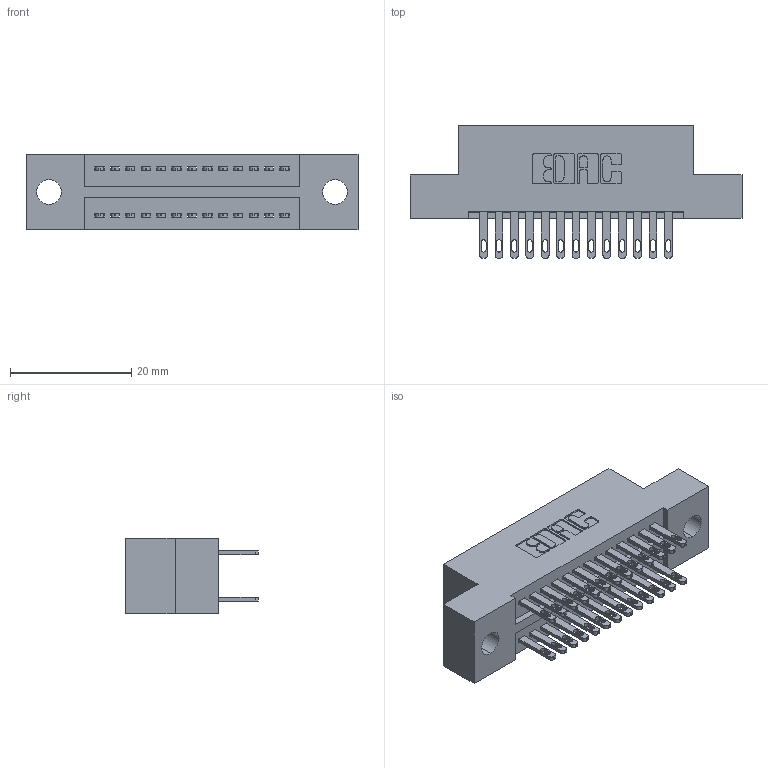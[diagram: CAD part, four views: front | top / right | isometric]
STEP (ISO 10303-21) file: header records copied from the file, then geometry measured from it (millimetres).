
FILE_DESCRIPTION (( 'STEP AP203' ), '1' );
FILE_NAME ('325-026-500-209.STEP', '2020-02-24T18:13:38', ( '' ), ( '' ), 'SwSTEP 2.0', 'SolidWorks 2016', '' );
FILE_SCHEMA (( 'CONFIG_CONTROL_DESIGN' ));
Length unit declared in the file: inch
Products named in the file (3): 325 Part_.160 TH; 325-292-001_325-293-100; 325-026-500-209
Assembly tree (27 placements, depth 2):
  325-026-500-209
    325 Part_.160 TH
    325-292-001_325-293-100  x26
Bounding box: 54.74 x 21.84 x 12.45 mm (x, y, z)
Volume: 6654.7 mm3; surface area: 7559.3 mm2
Topology: 27 solids, 27 shells, 1362 faces, 4133 edges, 2754 vertices
Faces by surface type: plane 850, cylinder 512
Entity records: 12047 total; most frequent: CARTESIAN_POINT 2030, ORIENTED_EDGE 1966, DIRECTION 1787, EDGE_CURVE 983, VECTOR 851, LINE 851, VERTEX_POINT 654, AXIS2_PLACEMENT_3D 468
